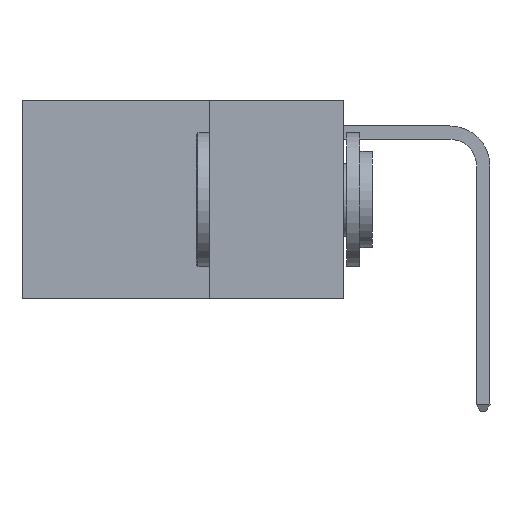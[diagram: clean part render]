
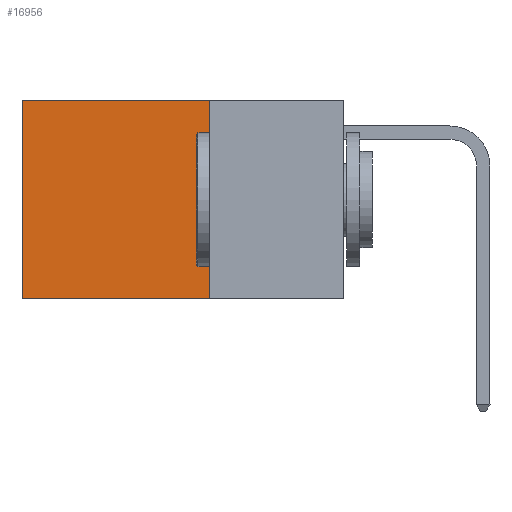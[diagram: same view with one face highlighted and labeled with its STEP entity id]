
A CAD part, left-side view. The second image highlights one B-rep face of the part: STEP entity #16956.
In plain terms, the highlighted planar face has unit normal (-1, 0, 0).
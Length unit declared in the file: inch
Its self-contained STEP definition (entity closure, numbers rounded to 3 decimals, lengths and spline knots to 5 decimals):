
#213 = DIRECTION ( 'NONE',  ( 0., 1., 0. ) ) ;
#791 = ORIENTED_EDGE ( 'NONE', *, *, #20833, .F. ) ;
#1045 = VECTOR ( 'NONE', #11572, 39.37008 ) ;
#1492 = DIRECTION ( 'NONE',  ( 0., 1., 0. ) ) ;
#2078 = VERTEX_POINT ( 'NONE', #15479 ) ;
#2478 = AXIS2_PLACEMENT_3D ( 'NONE', #5314, #22196, #11204 ) ;
#4680 = CARTESIAN_POINT ( 'NONE',  ( 0.2625, 0.25, -0.37 ) ) ;
#4904 = ORIENTED_EDGE ( 'NONE', *, *, #15873, .F. ) ;
#5042 = VERTEX_POINT ( 'NONE', #23333 ) ;
#5314 = CARTESIAN_POINT ( 'NONE',  ( 0.2625, 0.25, 0. ) ) ;
#6224 = LINE ( 'NONE', #15786, #22258 ) ;
#7340 = CARTESIAN_POINT ( 'NONE',  ( 0.2625, 0.25, -0.37 ) ) ;
#9256 = PLANE ( 'NONE',  #2478 ) ;
#9574 = ORIENTED_EDGE ( 'NONE', *, *, #15486, .T. ) ;
#11204 = DIRECTION ( 'NONE',  ( 0., 0., -1. ) ) ;
#11310 = LINE ( 'NONE', #15450, #1045 ) ;
#11572 = DIRECTION ( 'NONE',  ( 0., 0., -1. ) ) ;
#11905 = CARTESIAN_POINT ( 'NONE',  ( 0.2625, 0.25, 0. ) ) ;
#12150 = LINE ( 'NONE', #7340, #17124 ) ;
#12386 = VECTOR ( 'NONE', #213, 39.37008 ) ;
#14573 = VERTEX_POINT ( 'NONE', #4680 ) ;
#15450 = CARTESIAN_POINT ( 'NONE',  ( 0.2625, 0.25, 0. ) ) ;
#15479 = CARTESIAN_POINT ( 'NONE',  ( 0.2625, 0.25, 0. ) ) ;
#15486 = EDGE_CURVE ( 'NONE', #5042, #21025, #6224, .T. ) ;
#15786 = CARTESIAN_POINT ( 'NONE',  ( 0.2625, 0.6, 0. ) ) ;
#15873 = EDGE_CURVE ( 'NONE', #2078, #14573, #11310, .T. ) ;
#16956 = ADVANCED_FACE ( 'NONE', ( #23467 ), #9256, .F. ) ;
#17124 = VECTOR ( 'NONE', #1492, 39.37008 ) ;
#17286 = CARTESIAN_POINT ( 'NONE',  ( 0.2625, 0.6, -0.37 ) ) ;
#17346 = LINE ( 'NONE', #11905, #12386 ) ;
#17901 = ORIENTED_EDGE ( 'NONE', *, *, #22910, .T. ) ;
#19401 = DIRECTION ( 'NONE',  ( 0., 0., -1. ) ) ;
#20699 = EDGE_LOOP ( 'NONE', ( #9574, #791, #4904, #17901 ) ) ;
#20833 = EDGE_CURVE ( 'NONE', #14573, #21025, #12150, .T. ) ;
#21025 = VERTEX_POINT ( 'NONE', #17286 ) ;
#22196 = DIRECTION ( 'NONE',  ( 1., 0., 0. ) ) ;
#22258 = VECTOR ( 'NONE', #19401, 39.37008 ) ;
#22910 = EDGE_CURVE ( 'NONE', #2078, #5042, #17346, .T. ) ;
#23333 = CARTESIAN_POINT ( 'NONE',  ( 0.2625, 0.6, 0. ) ) ;
#23467 = FACE_OUTER_BOUND ( 'NONE', #20699, .T. ) ;
